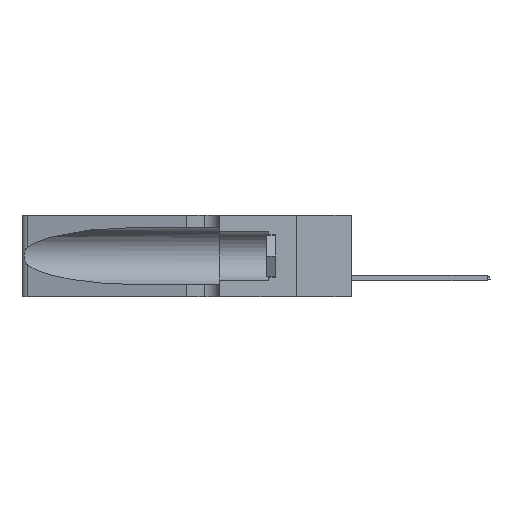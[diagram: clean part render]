
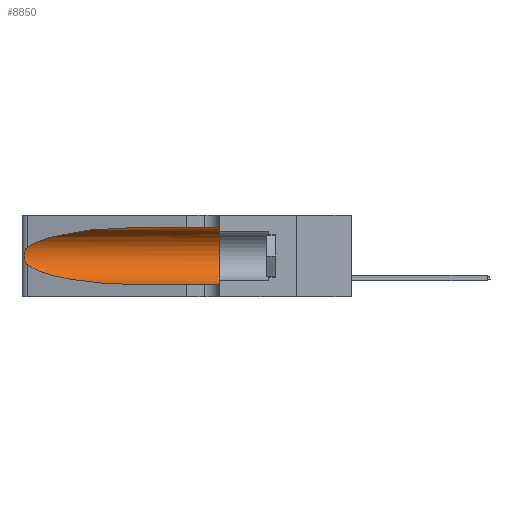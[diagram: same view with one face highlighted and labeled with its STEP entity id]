
A CAD part, left-side view. The second image highlights one B-rep face of the part: STEP entity #8850.
In plain terms, the highlighted cylindrical face has radius 3.308 mm (diameter 6.617 mm), a partial arc.
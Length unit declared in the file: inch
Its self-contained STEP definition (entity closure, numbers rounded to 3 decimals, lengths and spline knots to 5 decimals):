
#333 = DIRECTION ( 'NONE',  ( 0., -1., 0. ) ) ;
#1537 = EDGE_CURVE ( 'NONE', #25789, #26853, #6485, .T. ) ;
#2370 = CARTESIAN_POINT ( 'NONE',  ( 0.25639, 1.23184, 0.21858 ) ) ;
#2389 = CARTESIAN_POINT ( 'NONE',  ( 0.2373, 1.15595, 0.08982 ) ) ;
#3471 = CIRCLE ( 'NONE', #31295, 0.13025 ) ;
#3474 = CARTESIAN_POINT ( 'NONE',  ( 0.25487, 1.22718, 0.14631 ) ) ;
#4533 = CARTESIAN_POINT ( 'NONE',  ( 0.1305, 0.35, 0.185 ) ) ;
#4678 = CARTESIAN_POINT ( 'NONE',  ( 0.25487, 1.22718, 0.22369 ) ) ;
#5115 = CARTESIAN_POINT ( 'NONE',  ( 0.25787, 1.23484, 0.2124 ) ) ;
#5285 = VECTOR ( 'NONE', #23685, 39.37008 ) ;
#5367 = ORIENTED_EDGE ( 'NONE', *, *, #23535, .F. ) ;
#5541 = CARTESIAN_POINT ( 'NONE',  ( 0.25487, 1.22718, 0.14631 ) ) ;
#6449 = ORIENTED_EDGE ( 'NONE', *, *, #1537, .T. ) ;
#6485 = B_SPLINE_CURVE_WITH_KNOTS ( 'NONE', 3,
 ( #4678, #33423, #2370, #5115, #8272, #10929, #26121, #16060, #15850, #20869, #23601, #28995, #21094, #5541 ),
 .UNSPECIFIED., .F., .F.,
 ( 4, 2, 2, 2, 2, 2, 4 ),
 ( 0., 0.00027, 0.00053, 0.00107, 0.0016, 0.00187, 0.00214 ),
 .UNSPECIFIED. ) ;
#6852 = CARTESIAN_POINT ( 'NONE',  ( 0.1305, 0.72297, 0.31525 ) ) ;
#6978 = CYLINDRICAL_SURFACE ( 'NONE', #29406, 0.13025 ) ;
#7848 = ORIENTED_EDGE ( 'NONE', *, *, #17986, .T. ) ;
#8272 = CARTESIAN_POINT ( 'NONE',  ( 0.25854, 1.2359, 0.20912 ) ) ;
#8850 = ADVANCED_FACE ( 'NONE', ( #15584 ), #6978, .F. ) ;
#8936 = CARTESIAN_POINT ( 'NONE',  ( 0.25487, 1.22718, 0.22369 ) ) ;
#9271 = VERTEX_POINT ( 'NONE', #19141 ) ;
#10929 = CARTESIAN_POINT ( 'NONE',  ( 0.26018, 1.23835, 0.19895 ) ) ;
#11314 = EDGE_CURVE ( 'NONE', #17633, #25789, #32870, .T. ) ;
#12983 = VECTOR ( 'NONE', #21484, 39.37008 ) ;
#14898 = CARTESIAN_POINT ( 'NONE',  ( 0.1305, 0.35, 0.31525 ) ) ;
#15319 = CARTESIAN_POINT ( 'NONE',  ( 0.25487, 1.22718, 0.14631 ) ) ;
#15584 = FACE_OUTER_BOUND ( 'NONE', #30198, .T. ) ;
#15832 = VERTEX_POINT ( 'NONE', #14898 ) ;
#15850 = CARTESIAN_POINT ( 'NONE',  ( 0.26017, 1.23833, 0.17102 ) ) ;
#16060 = CARTESIAN_POINT ( 'NONE',  ( 0.26075, 1.23896, 0.178 ) ) ;
#16099 = EDGE_CURVE ( 'NONE', #15832, #22025, #3471, .T. ) ;
#16935 = CARTESIAN_POINT ( 'NONE',  ( 0.25487, 1.22718, 0.22369 ) ) ;
#17633 = VERTEX_POINT ( 'NONE', #6852 ) ;
#17734 = ORIENTED_EDGE ( 'NONE', *, *, #16099, .F. ) ;
#17986 = EDGE_CURVE ( 'NONE', #9271, #22025, #20393, .T. ) ;
#18282 = CARTESIAN_POINT ( 'NONE',  ( 0.1305, 0.72297, 0.05475 ) ) ;
#18600 = CARTESIAN_POINT ( 'NONE',  ( 0.1305, 1.61858, 0.185 ) ) ;
#19141 = CARTESIAN_POINT ( 'NONE',  ( 0.1305, 0.72297, 0.05475 ) ) ;
#20284 = EDGE_CURVE ( 'NONE', #26853, #9271, #26821, .T. ) ;
#20393 = LINE ( 'NONE', #26211, #5285 ) ;
#20869 = CARTESIAN_POINT ( 'NONE',  ( 0.25856, 1.23593, 0.16098 ) ) ;
#21094 = CARTESIAN_POINT ( 'NONE',  ( 0.25555, 1.22993, 0.14849 ) ) ;
#21484 = DIRECTION ( 'NONE',  ( 0., -1., 0. ) ) ;
#22025 = VERTEX_POINT ( 'NONE', #22288 ) ;
#22288 = CARTESIAN_POINT ( 'NONE',  ( 0.1305, 0.35, 0.05475 ) ) ;
#22645 = ORIENTED_EDGE ( 'NONE', *, *, #11314, .T. ) ;
#23535 = EDGE_CURVE ( 'NONE', #17633, #15832, #26887, .T. ) ;
#23601 = CARTESIAN_POINT ( 'NONE',  ( 0.25789, 1.23486, 0.15765 ) ) ;
#23685 = DIRECTION ( 'NONE',  ( 0., -1., 0. ) ) ;
#23943 = DIRECTION ( 'NONE',  ( 0., 0., -1. ) ) ;
#24071 = ORIENTED_EDGE ( 'NONE', *, *, #20284, .T. ) ;
#24966 = DIRECTION ( 'NONE',  ( 0., 1., 0. ) ) ;
#25789 = VERTEX_POINT ( 'NONE', #16935 ) ;
#25902 = CARTESIAN_POINT ( 'NONE',  ( 0.1305, 0.72297, 0.31525 ) ) ;
#26121 = CARTESIAN_POINT ( 'NONE',  ( 0.26075, 1.23896, 0.19203 ) ) ;
#26211 = CARTESIAN_POINT ( 'NONE',  ( 0.1305, 1.61858, 0.05475 ) ) ;
#26821 =( BOUNDED_CURVE ( )  B_SPLINE_CURVE ( 3, ( #15319, #2389, #28908, #18282 ),
 .UNSPECIFIED., .F., .F. ) 
 B_SPLINE_CURVE_WITH_KNOTS ( ( 4, 4 ),
 ( 3.44316, 4.71239 ),
 .UNSPECIFIED. ) 
 CURVE ( )  GEOMETRIC_REPRESENTATION_ITEM ( )  RATIONAL_B_SPLINE_CURVE ( ( 1., 0.87, 0.87, 1. ) ) 
 REPRESENTATION_ITEM ( '' )  );
#26853 = VERTEX_POINT ( 'NONE', #3474 ) ;
#26887 = LINE ( 'NONE', #29526, #12983 ) ;
#28908 = CARTESIAN_POINT ( 'NONE',  ( 0.18966, 0.96281, 0.05475 ) ) ;
#28995 = CARTESIAN_POINT ( 'NONE',  ( 0.25639, 1.23186, 0.15144 ) ) ;
#29406 = AXIS2_PLACEMENT_3D ( 'NONE', #18600, #333, #23943 ) ;
#29526 = CARTESIAN_POINT ( 'NONE',  ( 0.1305, 1.61858, 0.31525 ) ) ;
#30070 = CARTESIAN_POINT ( 'NONE',  ( 0.2373, 1.15595, 0.28018 ) ) ;
#30198 = EDGE_LOOP ( 'NONE', ( #22645, #6449, #24071, #7848, #17734, #5367 ) ) ;
#30350 = DIRECTION ( 'NONE',  ( 0., 0., 1. ) ) ;
#30416 = CARTESIAN_POINT ( 'NONE',  ( 0.18966, 0.96281, 0.31525 ) ) ;
#31295 = AXIS2_PLACEMENT_3D ( 'NONE', #4533, #24966, #30350 ) ;
#32870 =( BOUNDED_CURVE ( )  B_SPLINE_CURVE ( 3, ( #25902, #30416, #30070, #8936 ),
 .UNSPECIFIED., .F., .T. ) 
 B_SPLINE_CURVE_WITH_KNOTS ( ( 4, 4 ),
 ( 1.5708, 2.84003 ),
 .UNSPECIFIED. ) 
 CURVE ( )  GEOMETRIC_REPRESENTATION_ITEM ( )  RATIONAL_B_SPLINE_CURVE ( ( 1., 0.87, 0.87, 1. ) ) 
 REPRESENTATION_ITEM ( '' )  );
#33423 = CARTESIAN_POINT ( 'NONE',  ( 0.25555, 1.22994, 0.2215 ) ) ;
